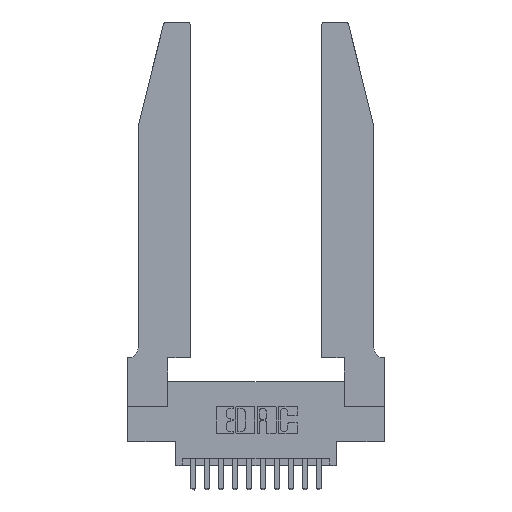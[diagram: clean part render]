
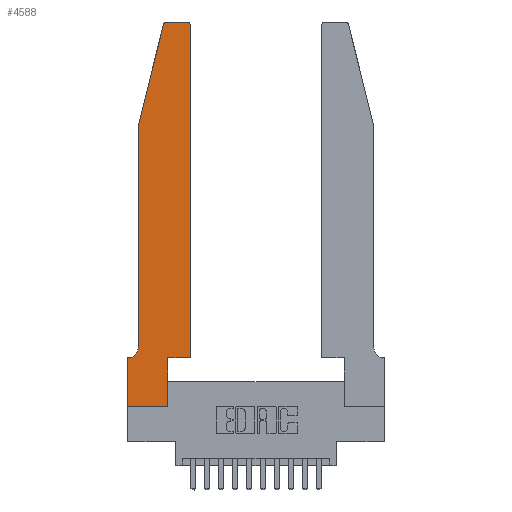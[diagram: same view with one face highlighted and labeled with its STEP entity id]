
A CAD part, top view. The second image highlights one B-rep face of the part: STEP entity #4588.
In plain terms, the highlighted planar face has unit normal (0, 0, 1).
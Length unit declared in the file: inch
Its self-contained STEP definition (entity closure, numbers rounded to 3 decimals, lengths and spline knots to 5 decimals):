
#48 = ORIENTED_EDGE ( 'NONE', *, *, #3574, .T. ) ;
#370 = DIRECTION ( 'NONE',  ( 1., 0., 0. ) ) ;
#377 = CIRCLE ( 'NONE', #5245, 0.07 ) ;
#586 = VECTOR ( 'NONE', #13225, 39.37008 ) ;
#846 = EDGE_CURVE ( 'NONE', #11732, #7730, #5108, .T. ) ;
#933 = CARTESIAN_POINT ( 'NONE',  ( 0.0755, 2., 0.37 ) ) ;
#1163 = VECTOR ( 'NONE', #2132, 39.37008 ) ;
#1187 = CARTESIAN_POINT ( 'NONE',  ( 0.25487, 2.72718, 0.37 ) ) ;
#1310 = ORIENTED_EDGE ( 'NONE', *, *, #11950, .T. ) ;
#1649 = ORIENTED_EDGE ( 'NONE', *, *, #5112, .T. ) ;
#1713 = CARTESIAN_POINT ( 'NONE',  ( 0.4205, 2.75, 0.37 ) ) ;
#1865 = DIRECTION ( 'NONE',  ( 1., 0., 0. ) ) ;
#1935 = AXIS2_PLACEMENT_3D ( 'NONE', #11196, #8673, #11298 ) ;
#2130 = CIRCLE ( 'NONE', #13947, 0.03 ) ;
#2132 = DIRECTION ( 'NONE',  ( 0., -1., 0. ) ) ;
#2154 = ORIENTED_EDGE ( 'NONE', *, *, #7017, .T. ) ;
#2355 = DIRECTION ( 'NONE',  ( -1., 0., 0. ) ) ;
#2686 = VERTEX_POINT ( 'NONE', #8303 ) ;
#2697 = VECTOR ( 'NONE', #1865, 39.37008 ) ;
#2939 = CARTESIAN_POINT ( 'NONE',  ( 0.0055, 0.35, 0.37 ) ) ;
#3149 = VERTEX_POINT ( 'NONE', #13674 ) ;
#3154 = VERTEX_POINT ( 'NONE', #2939 ) ;
#3574 = EDGE_CURVE ( 'NONE', #7730, #13935, #8681, .T. ) ;
#4136 = DIRECTION ( 'NONE',  ( -1., 0., 0. ) ) ;
#4436 = CARTESIAN_POINT ( 'NONE',  ( 0., 0., 0.37 ) ) ;
#4576 = CARTESIAN_POINT ( 'NONE',  ( 0.2865, 0.35, 0.37 ) ) ;
#4588 = ADVANCED_FACE ( 'NONE', ( #4881 ), #15239, .T. ) ;
#4605 = LINE ( 'NONE', #4576, #12878 ) ;
#4643 = VECTOR ( 'NONE', #4136, 39.37008 ) ;
#4881 = FACE_OUTER_BOUND ( 'NONE', #12530, .T. ) ;
#5108 = LINE ( 'NONE', #13016, #15252 ) ;
#5112 = EDGE_CURVE ( 'NONE', #15634, #11732, #2130, .T. ) ;
#5242 = DIRECTION ( 'NONE',  ( 0., 0., 1. ) ) ;
#5245 = AXIS2_PLACEMENT_3D ( 'NONE', #16928, #11463, #2355 ) ;
#5265 = CARTESIAN_POINT ( 'NONE',  ( 0.2865, 0., 0.37 ) ) ;
#5305 = CARTESIAN_POINT ( 'NONE',  ( 0.4205, 2.72, 0.37 ) ) ;
#5457 = VERTEX_POINT ( 'NONE', #5765 ) ;
#5639 = DIRECTION ( 'NONE',  ( 0., 1., 0. ) ) ;
#5657 = CARTESIAN_POINT ( 'NONE',  ( 0.284, 2.72, 0.37 ) ) ;
#5765 = CARTESIAN_POINT ( 'NONE',  ( 0., 0., 0.37 ) ) ;
#6030 = DIRECTION ( 'NONE',  ( 0., 1., 0. ) ) ;
#6775 = ORIENTED_EDGE ( 'NONE', *, *, #15145, .T. ) ;
#6955 = CARTESIAN_POINT ( 'NONE',  ( 0.4505, 2.72, 0.37 ) ) ;
#7017 = EDGE_CURVE ( 'NONE', #14427, #2686, #4605, .T. ) ;
#7134 = DIRECTION ( 'NONE',  ( 1., 0., 0. ) ) ;
#7223 = ORIENTED_EDGE ( 'NONE', *, *, #13511, .T. ) ;
#7730 = VERTEX_POINT ( 'NONE', #9072 ) ;
#8180 = CARTESIAN_POINT ( 'NONE',  ( 0.284, 2.75, 0.37 ) ) ;
#8303 = CARTESIAN_POINT ( 'NONE',  ( 0.2865, 0.35, 0.37 ) ) ;
#8673 = DIRECTION ( 'NONE',  ( 0., 0., 1. ) ) ;
#8681 = LINE ( 'NONE', #933, #1163 ) ;
#8810 = EDGE_CURVE ( 'NONE', #15851, #5457, #14074, .T. ) ;
#8992 = EDGE_CURVE ( 'NONE', #13935, #3154, #377, .T. ) ;
#9003 = ORIENTED_EDGE ( 'NONE', *, *, #846, .T. ) ;
#9037 = ORIENTED_EDGE ( 'NONE', *, *, #17159, .T. ) ;
#9072 = CARTESIAN_POINT ( 'NONE',  ( 0.0755, 2., 0.37 ) ) ;
#9317 = ORIENTED_EDGE ( 'NONE', *, *, #15840, .T. ) ;
#9352 = VECTOR ( 'NONE', #16410, 39.37008 ) ;
#10247 = ORIENTED_EDGE ( 'NONE', *, *, #8810, .T. ) ;
#10426 = LINE ( 'NONE', #4436, #2697 ) ;
#10468 = CARTESIAN_POINT ( 'NONE',  ( 0.0755, 0.35, 0.37 ) ) ;
#10946 = VECTOR ( 'NONE', #7134, 39.37008 ) ;
#10979 = CARTESIAN_POINT ( 'NONE',  ( 0.4505, 0.35, 0.37 ) ) ;
#11065 = CARTESIAN_POINT ( 'NONE',  ( 0.4505, 0.35, 0.37 ) ) ;
#11177 = LINE ( 'NONE', #10979, #14893 ) ;
#11196 = CARTESIAN_POINT ( 'NONE',  ( 0., 0.35, 0.37 ) ) ;
#11241 = EDGE_CURVE ( 'NONE', #15908, #12924, #15652, .T. ) ;
#11298 = DIRECTION ( 'NONE',  ( 1., 0., 0. ) ) ;
#11463 = DIRECTION ( 'NONE',  ( 0., 0., -1. ) ) ;
#11732 = VERTEX_POINT ( 'NONE', #1187 ) ;
#11950 = EDGE_CURVE ( 'NONE', #12924, #15634, #13334, .T. ) ;
#12031 = CARTESIAN_POINT ( 'NONE',  ( 0.2605, 2.75, 0.37 ) ) ;
#12374 = LINE ( 'NONE', #11065, #10946 ) ;
#12530 = EDGE_LOOP ( 'NONE', ( #1310, #1649, #9003, #48, #14362, #9037, #10247, #7223, #2154, #9317, #6775, #14518 ) ) ;
#12684 = AXIS2_PLACEMENT_3D ( 'NONE', #5305, #5242, #13377 ) ;
#12878 = VECTOR ( 'NONE', #6030, 39.37008 ) ;
#12924 = VERTEX_POINT ( 'NONE', #1713 ) ;
#13016 = CARTESIAN_POINT ( 'NONE',  ( 0.0755, 2., 0.37 ) ) ;
#13225 = DIRECTION ( 'NONE',  ( -1., 0., 0. ) ) ;
#13334 = LINE ( 'NONE', #12031, #4643 ) ;
#13377 = DIRECTION ( 'NONE',  ( 1., 0., 0. ) ) ;
#13511 = EDGE_CURVE ( 'NONE', #5457, #14427, #10426, .T. ) ;
#13674 = CARTESIAN_POINT ( 'NONE',  ( 0.4505, 0.35, 0.37 ) ) ;
#13771 = CARTESIAN_POINT ( 'NONE',  ( 0., 0.35, 0.37 ) ) ;
#13935 = VERTEX_POINT ( 'NONE', #14628 ) ;
#13947 = AXIS2_PLACEMENT_3D ( 'NONE', #5657, #14927, #370 ) ;
#14074 = LINE ( 'NONE', #15120, #9352 ) ;
#14331 = DIRECTION ( 'NONE',  ( -0.239, -0.971, 0. ) ) ;
#14362 = ORIENTED_EDGE ( 'NONE', *, *, #8992, .T. ) ;
#14427 = VERTEX_POINT ( 'NONE', #5265 ) ;
#14518 = ORIENTED_EDGE ( 'NONE', *, *, #11241, .T. ) ;
#14628 = CARTESIAN_POINT ( 'NONE',  ( 0.0755, 0.42, 0.37 ) ) ;
#14893 = VECTOR ( 'NONE', #5639, 39.37008 ) ;
#14927 = DIRECTION ( 'NONE',  ( 0., 0., 1. ) ) ;
#15115 = LINE ( 'NONE', #10468, #586 ) ;
#15120 = CARTESIAN_POINT ( 'NONE',  ( 0., 0., 0.37 ) ) ;
#15145 = EDGE_CURVE ( 'NONE', #3149, #15908, #11177, .T. ) ;
#15239 = PLANE ( 'NONE',  #1935 ) ;
#15252 = VECTOR ( 'NONE', #14331, 39.37008 ) ;
#15634 = VERTEX_POINT ( 'NONE', #8180 ) ;
#15652 = CIRCLE ( 'NONE', #12684, 0.03 ) ;
#15840 = EDGE_CURVE ( 'NONE', #2686, #3149, #12374, .T. ) ;
#15851 = VERTEX_POINT ( 'NONE', #13771 ) ;
#15908 = VERTEX_POINT ( 'NONE', #6955 ) ;
#16410 = DIRECTION ( 'NONE',  ( 0., -1., 0. ) ) ;
#16928 = CARTESIAN_POINT ( 'NONE',  ( 0.0055, 0.42, 0.37 ) ) ;
#17159 = EDGE_CURVE ( 'NONE', #3154, #15851, #15115, .T. ) ;
